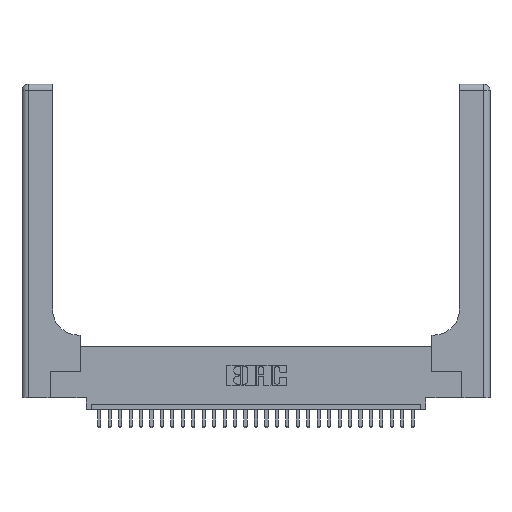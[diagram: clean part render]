
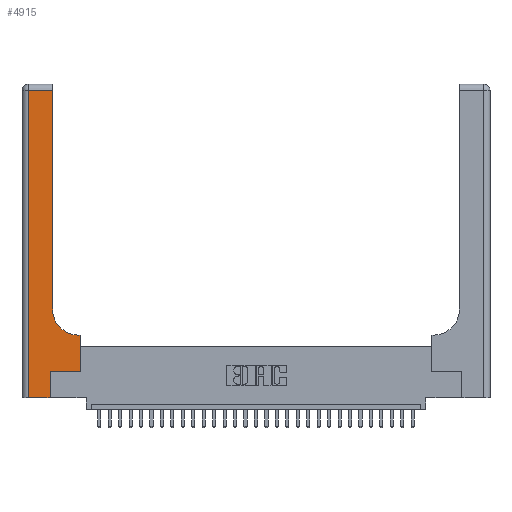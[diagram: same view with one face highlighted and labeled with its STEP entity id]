
A CAD part, top view. The second image highlights one B-rep face of the part: STEP entity #4915.
In plain terms, the highlighted planar face has unit normal (0, 0, 1).
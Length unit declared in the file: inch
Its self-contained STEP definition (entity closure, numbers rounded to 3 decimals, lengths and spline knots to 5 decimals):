
#17 = CARTESIAN_POINT ( 'NONE',  ( 0.5415, 0.6, 0.37 ) ) ;
#101 = CARTESIAN_POINT ( 'NONE',  ( 0.269, 0., 0.37 ) ) ;
#535 = ORIENTED_EDGE ( 'NONE', *, *, #27476, .T. ) ;
#1287 = DIRECTION ( 'NONE',  ( 0., 0., -1. ) ) ;
#1732 = DIRECTION ( 'NONE',  ( 1., 0., 0. ) ) ;
#2033 = LINE ( 'NONE', #3950, #9770 ) ;
#3286 = LINE ( 'NONE', #10493, #20519 ) ;
#3950 = CARTESIAN_POINT ( 'NONE',  ( 0., 2.94, 0.37 ) ) ;
#4915 = ADVANCED_FACE ( 'NONE', ( #14219 ), #10565, .F. ) ;
#5084 = ORIENTED_EDGE ( 'NONE', *, *, #18031, .T. ) ;
#7187 = VERTEX_POINT ( 'NONE', #15572 ) ;
#7489 = VERTEX_POINT ( 'NONE', #20749 ) ;
#8136 = CARTESIAN_POINT ( 'NONE',  ( 0.06, 3., 0.37 ) ) ;
#8869 = CARTESIAN_POINT ( 'NONE',  ( 0., 0., 0.37 ) ) ;
#9574 = CARTESIAN_POINT ( 'NONE',  ( 0.5585, 0.25, 0.37 ) ) ;
#9770 = VECTOR ( 'NONE', #11192, 39.37008 ) ;
#9795 = ORIENTED_EDGE ( 'NONE', *, *, #16140, .T. ) ;
#10493 = CARTESIAN_POINT ( 'NONE',  ( 0.2915, 3., 0.37 ) ) ;
#10557 = CIRCLE ( 'NONE', #25274, 0.25 ) ;
#10565 = PLANE ( 'NONE',  #26082 ) ;
#10603 = DIRECTION ( 'NONE',  ( 0., 1., 0. ) ) ;
#10992 = VECTOR ( 'NONE', #18282, 39.37008 ) ;
#11192 = DIRECTION ( 'NONE',  ( -1., 0., 0. ) ) ;
#12236 = ORIENTED_EDGE ( 'NONE', *, *, #17805, .T. ) ;
#12504 = DIRECTION ( 'NONE',  ( 0., -1., 0. ) ) ;
#12734 = CARTESIAN_POINT ( 'NONE',  ( 0., 3., 0.37 ) ) ;
#12784 = LINE ( 'NONE', #25034, #16048 ) ;
#13044 = DIRECTION ( 'NONE',  ( -1., 0., 0. ) ) ;
#13297 = CARTESIAN_POINT ( 'NONE',  ( 0.5415, 0.85, 0.37 ) ) ;
#13756 = LINE ( 'NONE', #8869, #19143 ) ;
#13980 = EDGE_CURVE ( 'NONE', #14787, #7187, #12784, .T. ) ;
#14196 = DIRECTION ( 'NONE',  ( 1., 0., 0. ) ) ;
#14219 = FACE_OUTER_BOUND ( 'NONE', #19292, .T. ) ;
#14468 = EDGE_CURVE ( 'NONE', #18655, #23161, #2033, .T. ) ;
#14787 = VERTEX_POINT ( 'NONE', #26885 ) ;
#15572 = CARTESIAN_POINT ( 'NONE',  ( 0.5585, 0.25, 0.37 ) ) ;
#15651 = LINE ( 'NONE', #8136, #17801 ) ;
#16048 = VECTOR ( 'NONE', #1732, 39.37008 ) ;
#16140 = EDGE_CURVE ( 'NONE', #26916, #29791, #13756, .T. ) ;
#16231 = DIRECTION ( 'NONE',  ( 0., 1., 0. ) ) ;
#17728 = DIRECTION ( 'NONE',  ( 0., 0., -1. ) ) ;
#17801 = VECTOR ( 'NONE', #12504, 39.37008 ) ;
#17805 = EDGE_CURVE ( 'NONE', #23161, #26916, #15651, .T. ) ;
#17967 = VECTOR ( 'NONE', #16231, 39.37008 ) ;
#18031 = EDGE_CURVE ( 'NONE', #29791, #14787, #20891, .T. ) ;
#18097 = ORIENTED_EDGE ( 'NONE', *, *, #29629, .T. ) ;
#18282 = DIRECTION ( 'NONE',  ( -1., 0., 0. ) ) ;
#18655 = VERTEX_POINT ( 'NONE', #20159 ) ;
#19097 = VERTEX_POINT ( 'NONE', #26846 ) ;
#19143 = VECTOR ( 'NONE', #14196, 39.37008 ) ;
#19292 = EDGE_LOOP ( 'NONE', ( #21498, #27741, #12236, #9795, #5084, #20047, #535, #18097, #25472 ) ) ;
#20047 = ORIENTED_EDGE ( 'NONE', *, *, #13980, .T. ) ;
#20159 = CARTESIAN_POINT ( 'NONE',  ( 0.2915, 2.94, 0.37 ) ) ;
#20519 = VECTOR ( 'NONE', #10603, 39.37008 ) ;
#20749 = CARTESIAN_POINT ( 'NONE',  ( 0.5585, 0.6, 0.37 ) ) ;
#20891 = LINE ( 'NONE', #29524, #26016 ) ;
#21200 = CARTESIAN_POINT ( 'NONE',  ( 0.06, 0., 0.37 ) ) ;
#21498 = ORIENTED_EDGE ( 'NONE', *, *, #27703, .T. ) ;
#22320 = DIRECTION ( 'NONE',  ( 1., 0., 0. ) ) ;
#22598 = CARTESIAN_POINT ( 'NONE',  ( 0.06, 2.94, 0.37 ) ) ;
#23161 = VERTEX_POINT ( 'NONE', #22598 ) ;
#23887 = VERTEX_POINT ( 'NONE', #17 ) ;
#24128 = LINE ( 'NONE', #9574, #17967 ) ;
#24424 = LINE ( 'NONE', #29537, #10992 ) ;
#24673 = DIRECTION ( 'NONE',  ( 0., 1., 0. ) ) ;
#25034 = CARTESIAN_POINT ( 'NONE',  ( 0.269, 0.25, 0.37 ) ) ;
#25274 = AXIS2_PLACEMENT_3D ( 'NONE', #13297, #17728, #22320 ) ;
#25472 = ORIENTED_EDGE ( 'NONE', *, *, #30154, .T. ) ;
#26016 = VECTOR ( 'NONE', #24673, 39.37008 ) ;
#26082 = AXIS2_PLACEMENT_3D ( 'NONE', #12734, #1287, #13044 ) ;
#26846 = CARTESIAN_POINT ( 'NONE',  ( 0.2915, 0.85, 0.37 ) ) ;
#26885 = CARTESIAN_POINT ( 'NONE',  ( 0.269, 0.25, 0.37 ) ) ;
#26916 = VERTEX_POINT ( 'NONE', #21200 ) ;
#27476 = EDGE_CURVE ( 'NONE', #7187, #7489, #24128, .T. ) ;
#27703 = EDGE_CURVE ( 'NONE', #19097, #18655, #3286, .T. ) ;
#27741 = ORIENTED_EDGE ( 'NONE', *, *, #14468, .T. ) ;
#29524 = CARTESIAN_POINT ( 'NONE',  ( 0.269, 0., 0.37 ) ) ;
#29537 = CARTESIAN_POINT ( 'NONE',  ( 0.2915, 0.6, 0.37 ) ) ;
#29629 = EDGE_CURVE ( 'NONE', #7489, #23887, #24424, .T. ) ;
#29791 = VERTEX_POINT ( 'NONE', #101 ) ;
#30154 = EDGE_CURVE ( 'NONE', #23887, #19097, #10557, .T. ) ;
